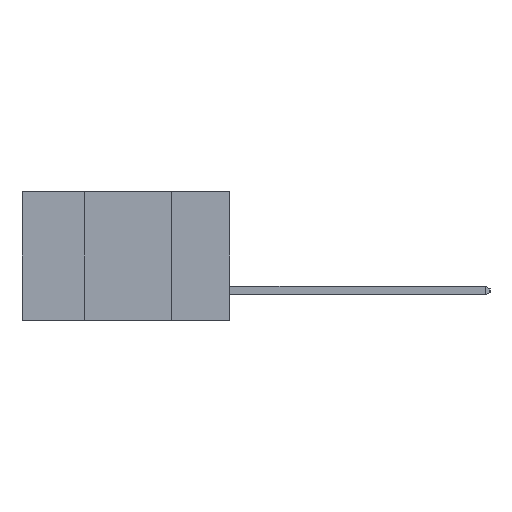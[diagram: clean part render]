
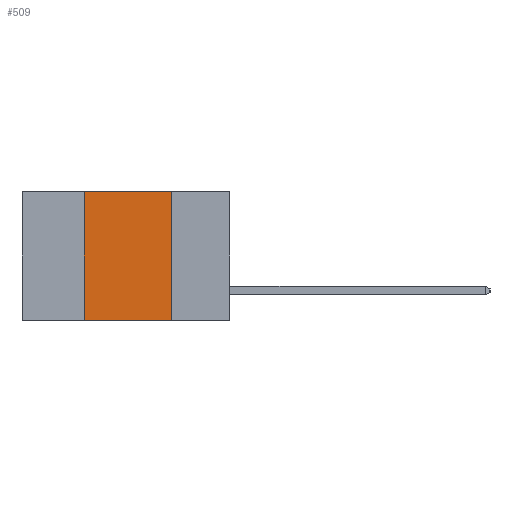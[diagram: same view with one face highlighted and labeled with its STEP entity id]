
A CAD part, left-side view. The second image highlights one B-rep face of the part: STEP entity #509.
In plain terms, the highlighted planar face has unit normal (-1, 0, 0).
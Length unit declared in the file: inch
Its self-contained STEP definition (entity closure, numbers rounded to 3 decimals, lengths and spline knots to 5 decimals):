
#509 = ADVANCED_FACE ( 'NONE', ( #22349 ), #2833, .F. ) ;
#1157 = VECTOR ( 'NONE', #22302, 39.37008 ) ;
#1673 = CARTESIAN_POINT ( 'NONE',  ( 0., 0.6, -0.37 ) ) ;
#2833 = PLANE ( 'NONE',  #4440 ) ;
#2857 = CARTESIAN_POINT ( 'NONE',  ( 0., 0.6, 0. ) ) ;
#3057 = DIRECTION ( 'NONE',  ( 0., 0., -1. ) ) ;
#3089 = DIRECTION ( 'NONE',  ( 1., 0., 0. ) ) ;
#3786 = VECTOR ( 'NONE', #21058, 39.37008 ) ;
#3897 = CARTESIAN_POINT ( 'NONE',  ( 0., 0.17, -0.37 ) ) ;
#3985 = DIRECTION ( 'NONE',  ( 0., 0., -1. ) ) ;
#4235 = VERTEX_POINT ( 'NONE', #16591 ) ;
#4440 = AXIS2_PLACEMENT_3D ( 'NONE', #2857, #3089, #3057 ) ;
#4741 = ORIENTED_EDGE ( 'NONE', *, *, #16172, .F. ) ;
#4972 = LINE ( 'NONE', #19210, #3786 ) ;
#8462 = VERTEX_POINT ( 'NONE', #21981 ) ;
#9354 = EDGE_CURVE ( 'NONE', #8462, #11055, #11194, .T. ) ;
#10400 = ORIENTED_EDGE ( 'NONE', *, *, #9354, .F. ) ;
#10898 = LINE ( 'NONE', #21200, #18451 ) ;
#11055 = VERTEX_POINT ( 'NONE', #14893 ) ;
#11194 = LINE ( 'NONE', #3897, #24111 ) ;
#11279 = LINE ( 'NONE', #1673, #1157 ) ;
#12312 = CARTESIAN_POINT ( 'NONE',  ( 0., 0.42, -0.37 ) ) ;
#13837 = DIRECTION ( 'NONE',  ( 0., -1., 0. ) ) ;
#14893 = CARTESIAN_POINT ( 'NONE',  ( 0., 0.17, -0.37 ) ) ;
#16172 = EDGE_CURVE ( 'NONE', #4235, #8462, #10898, .T. ) ;
#16591 = CARTESIAN_POINT ( 'NONE',  ( 0., 0.42, 0. ) ) ;
#17419 = VERTEX_POINT ( 'NONE', #12312 ) ;
#18451 = VECTOR ( 'NONE', #13837, 39.37008 ) ;
#18538 = ORIENTED_EDGE ( 'NONE', *, *, #20165, .T. ) ;
#19210 = CARTESIAN_POINT ( 'NONE',  ( 0., 0.42, -0.37 ) ) ;
#20165 = EDGE_CURVE ( 'NONE', #17419, #11055, #11279, .T. ) ;
#21058 = DIRECTION ( 'NONE',  ( 0., 0., 1. ) ) ;
#21200 = CARTESIAN_POINT ( 'NONE',  ( 0., 0.6, 0. ) ) ;
#21506 = EDGE_CURVE ( 'NONE', #17419, #4235, #4972, .T. ) ;
#21981 = CARTESIAN_POINT ( 'NONE',  ( 0., 0.17, 0. ) ) ;
#22302 = DIRECTION ( 'NONE',  ( 0., -1., 0. ) ) ;
#22349 = FACE_OUTER_BOUND ( 'NONE', #22779, .T. ) ;
#22779 = EDGE_LOOP ( 'NONE', ( #10400, #4741, #23357, #18538 ) ) ;
#23357 = ORIENTED_EDGE ( 'NONE', *, *, #21506, .F. ) ;
#24111 = VECTOR ( 'NONE', #3985, 39.37008 ) ;
